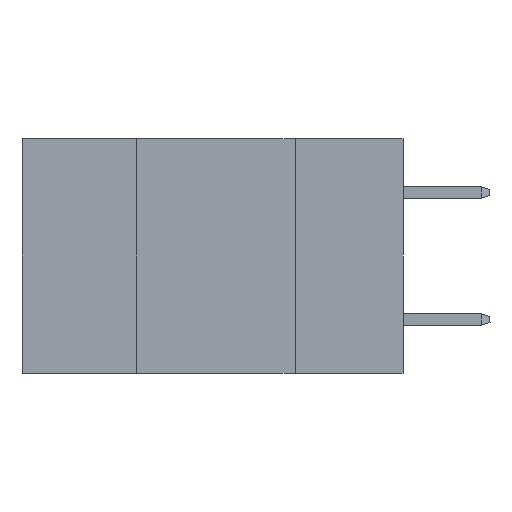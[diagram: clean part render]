
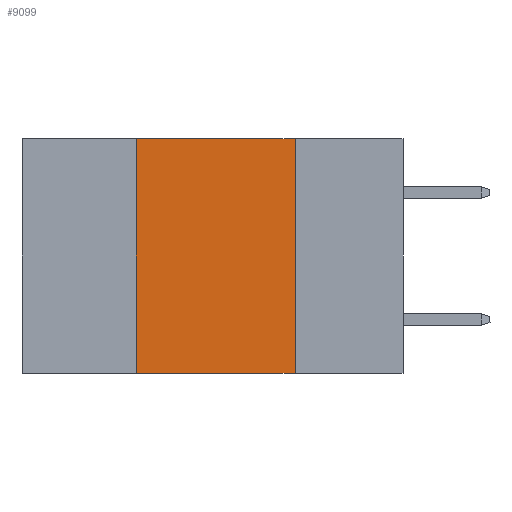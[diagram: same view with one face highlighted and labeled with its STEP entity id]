
A CAD part, left-side view. The second image highlights one B-rep face of the part: STEP entity #9099.
In plain terms, the highlighted planar face has unit normal (-1, 0, 0).
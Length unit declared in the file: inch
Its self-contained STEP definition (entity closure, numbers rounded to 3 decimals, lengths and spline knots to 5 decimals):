
#855 = CARTESIAN_POINT ( 'NONE',  ( 0., 0.6, 0. ) ) ;
#881 = LINE ( 'NONE', #11348, #2673 ) ;
#1259 = LINE ( 'NONE', #7556, #6784 ) ;
#1545 = EDGE_LOOP ( 'NONE', ( #8102, #7626, #3851, #12129 ) ) ;
#2673 = VECTOR ( 'NONE', #9225, 39.37008 ) ;
#3171 = CARTESIAN_POINT ( 'NONE',  ( 0., 0.6, -0.37 ) ) ;
#3851 = ORIENTED_EDGE ( 'NONE', *, *, #7235, .F. ) ;
#4492 = EDGE_CURVE ( 'NONE', #9927, #12824, #881, .T. ) ;
#5268 = LINE ( 'NONE', #3171, #13551 ) ;
#6376 = CARTESIAN_POINT ( 'NONE',  ( 0., 0.42, -0.37 ) ) ;
#6784 = VECTOR ( 'NONE', #12737, 39.37008 ) ;
#7235 = EDGE_CURVE ( 'NONE', #11620, #9698, #11398, .T. ) ;
#7255 = DIRECTION ( 'NONE',  ( 0., -1., 0. ) ) ;
#7556 = CARTESIAN_POINT ( 'NONE',  ( 0., 0.6, 0. ) ) ;
#7626 = ORIENTED_EDGE ( 'NONE', *, *, #12109, .F. ) ;
#7796 = EDGE_CURVE ( 'NONE', #11620, #12824, #5268, .T. ) ;
#7900 = CARTESIAN_POINT ( 'NONE',  ( 0., 0.42, 0. ) ) ;
#8102 = ORIENTED_EDGE ( 'NONE', *, *, #4492, .F. ) ;
#8247 = PLANE ( 'NONE',  #9564 ) ;
#9099 = ADVANCED_FACE ( 'NONE', ( #10276 ), #8247, .F. ) ;
#9225 = DIRECTION ( 'NONE',  ( 0., 0., -1. ) ) ;
#9269 = CARTESIAN_POINT ( 'NONE',  ( 0., 0.42, 0. ) ) ;
#9564 = AXIS2_PLACEMENT_3D ( 'NONE', #855, #12399, #11452 ) ;
#9698 = VERTEX_POINT ( 'NONE', #7900 ) ;
#9927 = VERTEX_POINT ( 'NONE', #11434 ) ;
#10276 = FACE_OUTER_BOUND ( 'NONE', #1545, .T. ) ;
#10359 = DIRECTION ( 'NONE',  ( 0., 0., 1. ) ) ;
#11348 = CARTESIAN_POINT ( 'NONE',  ( 0., 0.17, 0. ) ) ;
#11398 = LINE ( 'NONE', #9269, #12001 ) ;
#11434 = CARTESIAN_POINT ( 'NONE',  ( 0., 0.17, 0. ) ) ;
#11452 = DIRECTION ( 'NONE',  ( 0., 0., -1. ) ) ;
#11620 = VERTEX_POINT ( 'NONE', #6376 ) ;
#12001 = VECTOR ( 'NONE', #10359, 39.37008 ) ;
#12109 = EDGE_CURVE ( 'NONE', #9698, #9927, #1259, .T. ) ;
#12129 = ORIENTED_EDGE ( 'NONE', *, *, #7796, .T. ) ;
#12399 = DIRECTION ( 'NONE',  ( 1., 0., 0. ) ) ;
#12681 = CARTESIAN_POINT ( 'NONE',  ( 0., 0.17, -0.37 ) ) ;
#12737 = DIRECTION ( 'NONE',  ( 0., -1., 0. ) ) ;
#12824 = VERTEX_POINT ( 'NONE', #12681 ) ;
#13551 = VECTOR ( 'NONE', #7255, 39.37008 ) ;
